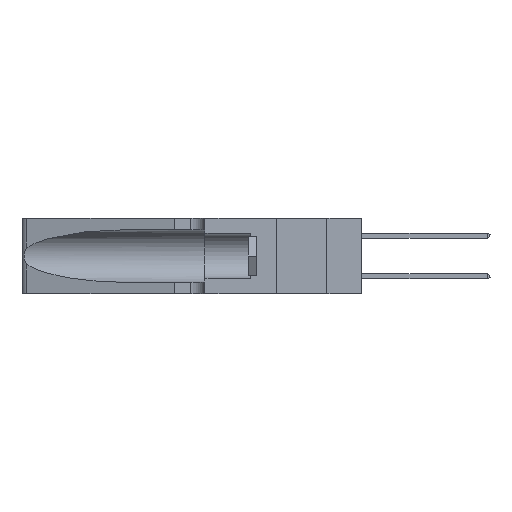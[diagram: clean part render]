
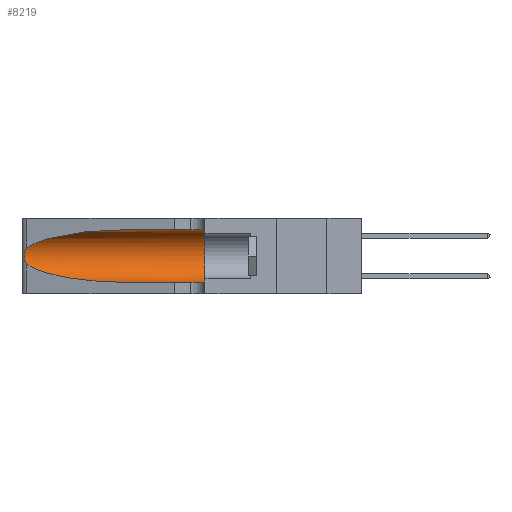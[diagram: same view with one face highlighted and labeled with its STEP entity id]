
A CAD part, left-side view. The second image highlights one B-rep face of the part: STEP entity #8219.
In plain terms, the highlighted cylindrical face has radius 3.308 mm (diameter 6.617 mm), a partial arc.
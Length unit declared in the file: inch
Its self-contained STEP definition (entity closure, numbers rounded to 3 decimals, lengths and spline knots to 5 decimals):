
#563 = CIRCLE ( 'NONE', #2948, 0.13025 ) ;
#696 = CARTESIAN_POINT ( 'NONE',  ( 0.25787, 1.23484, 0.2124 ) ) ;
#1035 = EDGE_CURVE ( 'NONE', #22329, #20544, #9503, .T. ) ;
#1903 = CARTESIAN_POINT ( 'NONE',  ( 0.25639, 1.23186, 0.15144 ) ) ;
#2110 = CARTESIAN_POINT ( 'NONE',  ( 0.26018, 1.23835, 0.19895 ) ) ;
#2133 = CARTESIAN_POINT ( 'NONE',  ( 0.25487, 1.22718, 0.22369 ) ) ;
#2463 = CARTESIAN_POINT ( 'NONE',  ( 0.26017, 1.23833, 0.17102 ) ) ;
#2489 = CARTESIAN_POINT ( 'NONE',  ( 0.25854, 1.2359, 0.20912 ) ) ;
#2498 = CARTESIAN_POINT ( 'NONE',  ( 0.25487, 1.22718, 0.14631 ) ) ;
#2527 = VERTEX_POINT ( 'NONE', #2634 ) ;
#2634 = CARTESIAN_POINT ( 'NONE',  ( 0.1305, 0.35, 0.31525 ) ) ;
#2731 = CARTESIAN_POINT ( 'NONE',  ( 0.25555, 1.22994, 0.2215 ) ) ;
#2948 = AXIS2_PLACEMENT_3D ( 'NONE', #3270, #15889, #5095 ) ;
#3270 = CARTESIAN_POINT ( 'NONE',  ( 0.1305, 0.35, 0.185 ) ) ;
#3455 = FACE_OUTER_BOUND ( 'NONE', #12653, .T. ) ;
#3704 = EDGE_CURVE ( 'NONE', #20544, #11185, #19954, .T. ) ;
#4050 = CARTESIAN_POINT ( 'NONE',  ( 0.25856, 1.23593, 0.16098 ) ) ;
#4108 = CARTESIAN_POINT ( 'NONE',  ( 0.25789, 1.23486, 0.15765 ) ) ;
#4448 = ORIENTED_EDGE ( 'NONE', *, *, #5380, .T. ) ;
#4690 = EDGE_CURVE ( 'NONE', #11185, #7490, #13902, .T. ) ;
#4878 = CARTESIAN_POINT ( 'NONE',  ( 0.26075, 1.23896, 0.19203 ) ) ;
#4929 = CARTESIAN_POINT ( 'NONE',  ( 0.25487, 1.22718, 0.14631 ) ) ;
#5095 = DIRECTION ( 'NONE',  ( 0., 0., 1. ) ) ;
#5380 = EDGE_CURVE ( 'NONE', #10718, #22329, #15999, .T. ) ;
#5543 = CARTESIAN_POINT ( 'NONE',  ( 0.1305, 0.72297, 0.31525 ) ) ;
#6189 = CARTESIAN_POINT ( 'NONE',  ( 0.1305, 0.72297, 0.05475 ) ) ;
#6219 = ORIENTED_EDGE ( 'NONE', *, *, #4690, .T. ) ;
#7066 = ORIENTED_EDGE ( 'NONE', *, *, #3704, .T. ) ;
#7490 = VERTEX_POINT ( 'NONE', #14776 ) ;
#7633 = CARTESIAN_POINT ( 'NONE',  ( 0.26075, 1.23896, 0.178 ) ) ;
#7659 = CARTESIAN_POINT ( 'NONE',  ( 0.25555, 1.22993, 0.14849 ) ) ;
#7732 = DIRECTION ( 'NONE',  ( 0., 0., -1. ) ) ;
#7927 = ORIENTED_EDGE ( 'NONE', *, *, #1035, .T. ) ;
#7968 = VECTOR ( 'NONE', #21012, 39.37008 ) ;
#8006 = AXIS2_PLACEMENT_3D ( 'NONE', #18305, #16585, #7732 ) ;
#8219 = ADVANCED_FACE ( 'NONE', ( #3455 ), #17190, .F. ) ;
#9286 = CARTESIAN_POINT ( 'NONE',  ( 0.2373, 1.15595, 0.28018 ) ) ;
#9346 = EDGE_CURVE ( 'NONE', #2527, #7490, #563, .T. ) ;
#9503 = B_SPLINE_CURVE_WITH_KNOTS ( 'NONE', 3,
 ( #2133, #2731, #21884, #696, #2489, #2110, #4878, #7633, #2463, #4050, #4108, #1903, #7659, #4929 ),
 .UNSPECIFIED., .F., .F.,
 ( 4, 2, 2, 2, 2, 2, 4 ),
 ( 0., 0.00027, 0.00053, 0.00107, 0.0016, 0.00187, 0.00214 ),
 .UNSPECIFIED. ) ;
#10718 = VERTEX_POINT ( 'NONE', #19553 ) ;
#10775 = DIRECTION ( 'NONE',  ( 0., -1., 0. ) ) ;
#11185 = VERTEX_POINT ( 'NONE', #20651 ) ;
#12077 = VECTOR ( 'NONE', #10775, 39.37008 ) ;
#12653 = EDGE_LOOP ( 'NONE', ( #4448, #7927, #7066, #6219, #13885, #15790 ) ) ;
#13433 = CARTESIAN_POINT ( 'NONE',  ( 0.2373, 1.15595, 0.08982 ) ) ;
#13885 = ORIENTED_EDGE ( 'NONE', *, *, #9346, .F. ) ;
#13902 = LINE ( 'NONE', #14205, #7968 ) ;
#14205 = CARTESIAN_POINT ( 'NONE',  ( 0.1305, 1.61858, 0.05475 ) ) ;
#14327 = CARTESIAN_POINT ( 'NONE',  ( 0.25487, 1.22718, 0.14631 ) ) ;
#14333 = CARTESIAN_POINT ( 'NONE',  ( 0.25487, 1.22718, 0.22369 ) ) ;
#14776 = CARTESIAN_POINT ( 'NONE',  ( 0.1305, 0.35, 0.05475 ) ) ;
#15790 = ORIENTED_EDGE ( 'NONE', *, *, #17286, .F. ) ;
#15889 = DIRECTION ( 'NONE',  ( 0., 1., 0. ) ) ;
#15999 =( BOUNDED_CURVE ( )  B_SPLINE_CURVE ( 3, ( #5543, #16295, #9286, #21423 ),
 .UNSPECIFIED., .F., .F. ) 
 B_SPLINE_CURVE_WITH_KNOTS ( ( 4, 4 ),
 ( 1.5708, 2.84003 ),
 .UNSPECIFIED. ) 
 CURVE ( )  GEOMETRIC_REPRESENTATION_ITEM ( )  RATIONAL_B_SPLINE_CURVE ( ( 1., 0.87, 0.87, 1. ) ) 
 REPRESENTATION_ITEM ( '' )  );
#16295 = CARTESIAN_POINT ( 'NONE',  ( 0.18966, 0.96281, 0.31525 ) ) ;
#16585 = DIRECTION ( 'NONE',  ( 0., -1., 0. ) ) ;
#16886 = CARTESIAN_POINT ( 'NONE',  ( 0.18966, 0.96281, 0.05475 ) ) ;
#17190 = CYLINDRICAL_SURFACE ( 'NONE', #8006, 0.13025 ) ;
#17286 = EDGE_CURVE ( 'NONE', #10718, #2527, #21155, .T. ) ;
#18305 = CARTESIAN_POINT ( 'NONE',  ( 0.1305, 1.61858, 0.185 ) ) ;
#19553 = CARTESIAN_POINT ( 'NONE',  ( 0.1305, 0.72297, 0.31525 ) ) ;
#19954 =( BOUNDED_CURVE ( )  B_SPLINE_CURVE ( 3, ( #2498, #13433, #16886, #6189 ),
 .UNSPECIFIED., .F., .F. ) 
 B_SPLINE_CURVE_WITH_KNOTS ( ( 4, 4 ),
 ( 3.44316, 4.71239 ),
 .UNSPECIFIED. ) 
 CURVE ( )  GEOMETRIC_REPRESENTATION_ITEM ( )  RATIONAL_B_SPLINE_CURVE ( ( 1., 0.87, 0.87, 1. ) ) 
 REPRESENTATION_ITEM ( '' )  );
#20544 = VERTEX_POINT ( 'NONE', #14327 ) ;
#20651 = CARTESIAN_POINT ( 'NONE',  ( 0.1305, 0.72297, 0.05475 ) ) ;
#21012 = DIRECTION ( 'NONE',  ( 0., -1., 0. ) ) ;
#21066 = CARTESIAN_POINT ( 'NONE',  ( 0.1305, 1.61858, 0.31525 ) ) ;
#21155 = LINE ( 'NONE', #21066, #12077 ) ;
#21423 = CARTESIAN_POINT ( 'NONE',  ( 0.25487, 1.22718, 0.22369 ) ) ;
#21884 = CARTESIAN_POINT ( 'NONE',  ( 0.25639, 1.23184, 0.21858 ) ) ;
#22329 = VERTEX_POINT ( 'NONE', #14333 ) ;
